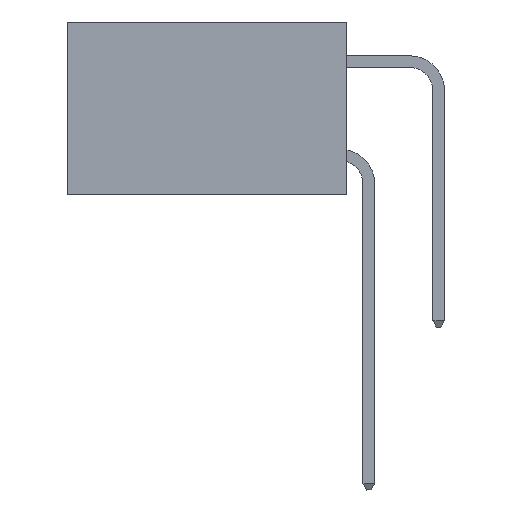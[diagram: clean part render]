
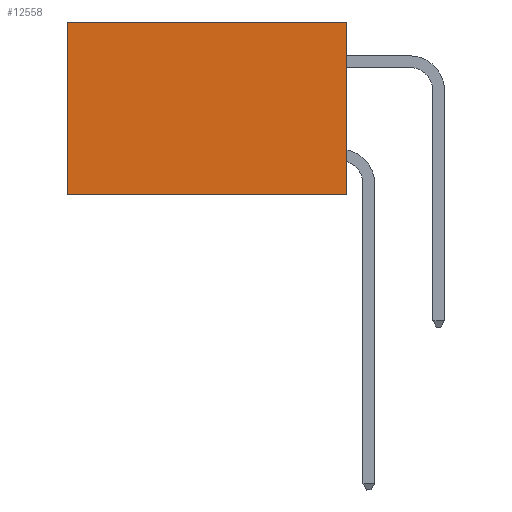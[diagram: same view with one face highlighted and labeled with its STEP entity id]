
A CAD part, left-side view. The second image highlights one B-rep face of the part: STEP entity #12558.
In plain terms, the highlighted planar face has unit normal (-1, 0, 0).
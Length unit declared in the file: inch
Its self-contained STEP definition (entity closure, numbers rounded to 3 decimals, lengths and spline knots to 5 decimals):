
#658 = CARTESIAN_POINT ( 'NONE',  ( 0.2875, 0., 0. ) ) ;
#1409 = LINE ( 'NONE', #36673, #20011 ) ;
#2681 = EDGE_CURVE ( 'NONE', #2826, #32654, #23233, .T. ) ;
#2826 = VERTEX_POINT ( 'NONE', #658 ) ;
#3939 = EDGE_CURVE ( 'NONE', #32654, #32572, #1409, .T. ) ;
#4944 = ORIENTED_EDGE ( 'NONE', *, *, #3939, .T. ) ;
#5507 = VERTEX_POINT ( 'NONE', #31571 ) ;
#6391 = CARTESIAN_POINT ( 'NONE',  ( 0.2875, 0., 0. ) ) ;
#8815 = ORIENTED_EDGE ( 'NONE', *, *, #11284, .F. ) ;
#9695 = AXIS2_PLACEMENT_3D ( 'NONE', #6391, #15246, #26689 ) ;
#10835 = EDGE_LOOP ( 'NONE', ( #4944, #17212, #8815, #12348 ) ) ;
#11284 = EDGE_CURVE ( 'NONE', #2826, #5507, #11637, .T. ) ;
#11491 = LINE ( 'NONE', #24112, #26022 ) ;
#11637 = LINE ( 'NONE', #23225, #16195 ) ;
#12348 = ORIENTED_EDGE ( 'NONE', *, *, #2681, .T. ) ;
#12558 = ADVANCED_FACE ( 'NONE', ( #19279 ), #14984, .F. ) ;
#14984 = PLANE ( 'NONE',  #9695 ) ;
#15234 = CARTESIAN_POINT ( 'NONE',  ( 0.2875, 0.6, -0.37 ) ) ;
#15246 = DIRECTION ( 'NONE',  ( 1., 0., 0. ) ) ;
#15478 = CARTESIAN_POINT ( 'NONE',  ( 0.2875, 0.6, 0. ) ) ;
#16195 = VECTOR ( 'NONE', #20510, 39.37008 ) ;
#17212 = ORIENTED_EDGE ( 'NONE', *, *, #28443, .F. ) ;
#19279 = FACE_OUTER_BOUND ( 'NONE', #10835, .T. ) ;
#20011 = VECTOR ( 'NONE', #21774, 39.37008 ) ;
#20510 = DIRECTION ( 'NONE',  ( 0., 0., -1. ) ) ;
#21378 = VECTOR ( 'NONE', #22521, 39.37008 ) ;
#21671 = DIRECTION ( 'NONE',  ( 0., 1., 0. ) ) ;
#21774 = DIRECTION ( 'NONE',  ( 0., 0., -1. ) ) ;
#22521 = DIRECTION ( 'NONE',  ( 0., 1., 0. ) ) ;
#23225 = CARTESIAN_POINT ( 'NONE',  ( 0.2875, 0., 0. ) ) ;
#23233 = LINE ( 'NONE', #33940, #21378 ) ;
#24112 = CARTESIAN_POINT ( 'NONE',  ( 0.2875, 0., -0.37 ) ) ;
#26022 = VECTOR ( 'NONE', #21671, 39.37008 ) ;
#26689 = DIRECTION ( 'NONE',  ( 0., 0., -1. ) ) ;
#28443 = EDGE_CURVE ( 'NONE', #5507, #32572, #11491, .T. ) ;
#31571 = CARTESIAN_POINT ( 'NONE',  ( 0.2875, 0., -0.37 ) ) ;
#32572 = VERTEX_POINT ( 'NONE', #15234 ) ;
#32654 = VERTEX_POINT ( 'NONE', #15478 ) ;
#33940 = CARTESIAN_POINT ( 'NONE',  ( 0.2875, 0., 0. ) ) ;
#36673 = CARTESIAN_POINT ( 'NONE',  ( 0.2875, 0.6, 0. ) ) ;
